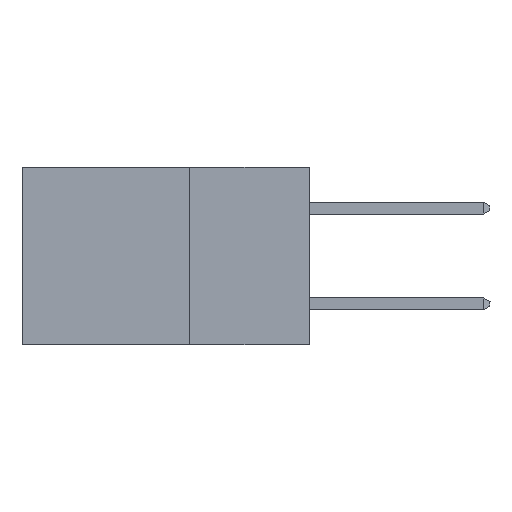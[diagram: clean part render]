
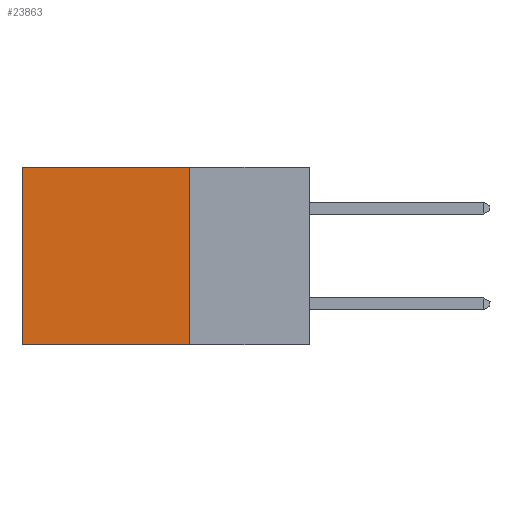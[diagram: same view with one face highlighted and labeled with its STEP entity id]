
A CAD part, left-side view. The second image highlights one B-rep face of the part: STEP entity #23863.
In plain terms, the highlighted planar face has unit normal (-1, 0, 0).
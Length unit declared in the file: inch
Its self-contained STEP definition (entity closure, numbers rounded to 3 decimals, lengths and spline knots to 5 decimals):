
#1608 = DIRECTION ( 'NONE',  ( 1., 0., 0. ) ) ;
#2018 = LINE ( 'NONE', #12052, #35332 ) ;
#2549 = CARTESIAN_POINT ( 'NONE',  ( 0.2875, 0.6, 0. ) ) ;
#2794 = ORIENTED_EDGE ( 'NONE', *, *, #35311, .F. ) ;
#3905 = DIRECTION ( 'NONE',  ( 0., 1., 0. ) ) ;
#4381 = FACE_OUTER_BOUND ( 'NONE', #22446, .T. ) ;
#4469 = CARTESIAN_POINT ( 'NONE',  ( 0.2875, 0.25, -0.37 ) ) ;
#6164 = LINE ( 'NONE', #12072, #35071 ) ;
#6304 = VECTOR ( 'NONE', #24711, 39.37008 ) ;
#7652 = CARTESIAN_POINT ( 'NONE',  ( 0.2875, 0.25, 0. ) ) ;
#7667 = AXIS2_PLACEMENT_3D ( 'NONE', #26949, #1608, #13000 ) ;
#9981 = CARTESIAN_POINT ( 'NONE',  ( 0.2875, 0.25, 0. ) ) ;
#10067 = ORIENTED_EDGE ( 'NONE', *, *, #24123, .F. ) ;
#11352 = VERTEX_POINT ( 'NONE', #4469 ) ;
#11763 = VECTOR ( 'NONE', #28173, 39.37008 ) ;
#12052 = CARTESIAN_POINT ( 'NONE',  ( 0.2875, 0.6, 0. ) ) ;
#12072 = CARTESIAN_POINT ( 'NONE',  ( 0.2875, 0.25, 0. ) ) ;
#13000 = DIRECTION ( 'NONE',  ( 0., 0., -1. ) ) ;
#14976 = VERTEX_POINT ( 'NONE', #22040 ) ;
#16865 = CARTESIAN_POINT ( 'NONE',  ( 0.2875, 0.25, -0.37 ) ) ;
#20265 = ORIENTED_EDGE ( 'NONE', *, *, #28978, .T. ) ;
#22040 = CARTESIAN_POINT ( 'NONE',  ( 0.2875, 0.6, -0.37 ) ) ;
#22446 = EDGE_LOOP ( 'NONE', ( #29730, #10067, #2794, #20265 ) ) ;
#22975 = EDGE_CURVE ( 'NONE', #31504, #14976, #2018, .T. ) ;
#23863 = ADVANCED_FACE ( 'NONE', ( #4381 ), #29298, .F. ) ;
#24123 = EDGE_CURVE ( 'NONE', #11352, #14976, #26669, .T. ) ;
#24711 = DIRECTION ( 'NONE',  ( 0., 0., -1. ) ) ;
#26669 = LINE ( 'NONE', #16865, #11763 ) ;
#26949 = CARTESIAN_POINT ( 'NONE',  ( 0.2875, 0.25, 0. ) ) ;
#28173 = DIRECTION ( 'NONE',  ( 0., 1., 0. ) ) ;
#28613 = DIRECTION ( 'NONE',  ( 0., 0., -1. ) ) ;
#28978 = EDGE_CURVE ( 'NONE', #33356, #31504, #6164, .T. ) ;
#29298 = PLANE ( 'NONE',  #7667 ) ;
#29730 = ORIENTED_EDGE ( 'NONE', *, *, #22975, .T. ) ;
#31504 = VERTEX_POINT ( 'NONE', #2549 ) ;
#33356 = VERTEX_POINT ( 'NONE', #7652 ) ;
#35071 = VECTOR ( 'NONE', #3905, 39.37008 ) ;
#35311 = EDGE_CURVE ( 'NONE', #33356, #11352, #36093, .T. ) ;
#35332 = VECTOR ( 'NONE', #28613, 39.37008 ) ;
#36093 = LINE ( 'NONE', #9981, #6304 ) ;
